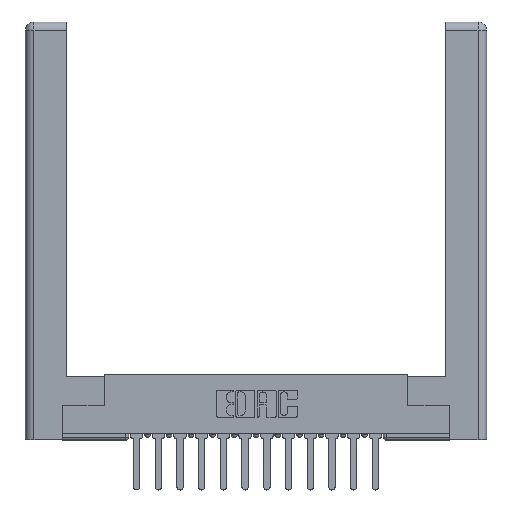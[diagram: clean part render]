
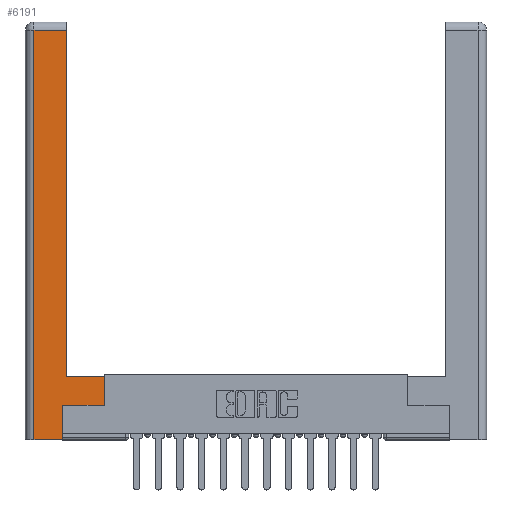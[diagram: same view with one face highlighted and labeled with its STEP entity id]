
A CAD part, top view. The second image highlights one B-rep face of the part: STEP entity #6191.
In plain terms, the highlighted planar face has unit normal (0, 0, 1).
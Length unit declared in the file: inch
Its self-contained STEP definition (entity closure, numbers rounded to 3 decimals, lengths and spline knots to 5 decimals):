
#5 = DIRECTION ( 'NONE',  ( -1., 0., 0. ) ) ;
#733 = LINE ( 'NONE', #2694, #1155 ) ;
#1034 = CARTESIAN_POINT ( 'NONE',  ( 0.565, 0.245, 0. ) ) ;
#1141 = DIRECTION ( 'NONE',  ( -1., 0., 0. ) ) ;
#1155 = VECTOR ( 'NONE', #15432, 39.37008 ) ;
#1436 = LINE ( 'NONE', #6506, #6390 ) ;
#1585 = VERTEX_POINT ( 'NONE', #7321 ) ;
#1708 = EDGE_CURVE ( 'NONE', #6962, #1585, #14943, .T. ) ;
#2441 = VERTEX_POINT ( 'NONE', #6844 ) ;
#2444 = CARTESIAN_POINT ( 'NONE',  ( 0.265, 0.245, 0. ) ) ;
#2694 = CARTESIAN_POINT ( 'NONE',  ( 0.295, 3., 0. ) ) ;
#2912 = EDGE_CURVE ( 'NONE', #2441, #9226, #13292, .T. ) ;
#3000 = CARTESIAN_POINT ( 'NONE',  ( 0.265, 0., 0. ) ) ;
#3029 = EDGE_CURVE ( 'NONE', #1585, #14190, #6334, .T. ) ;
#3034 = CARTESIAN_POINT ( 'NONE',  ( 0.565, 0.45, 0. ) ) ;
#3128 = LINE ( 'NONE', #3000, #5812 ) ;
#3150 = EDGE_CURVE ( 'NONE', #5322, #2441, #16774, .T. ) ;
#4112 = EDGE_CURVE ( 'NONE', #9226, #6962, #733, .T. ) ;
#4946 = CARTESIAN_POINT ( 'NONE',  ( 0.295, 0.45, 0. ) ) ;
#5085 = VECTOR ( 'NONE', #12213, 39.37008 ) ;
#5322 = VERTEX_POINT ( 'NONE', #12690 ) ;
#5392 = CARTESIAN_POINT ( 'NONE',  ( 0.0615, 2.94, 0. ) ) ;
#5812 = VECTOR ( 'NONE', #12168, 39.37008 ) ;
#6191 = ADVANCED_FACE ( 'NONE', ( #7408 ), #15549, .F. ) ;
#6334 = LINE ( 'NONE', #15908, #10617 ) ;
#6390 = VECTOR ( 'NONE', #15738, 39.37008 ) ;
#6506 = CARTESIAN_POINT ( 'NONE',  ( 0.265, 0.245, 0. ) ) ;
#6844 = CARTESIAN_POINT ( 'NONE',  ( 0.565, 0.45, 0. ) ) ;
#6962 = VERTEX_POINT ( 'NONE', #15810 ) ;
#7321 = CARTESIAN_POINT ( 'NONE',  ( 0.0615, 2.94, 0. ) ) ;
#7379 = ORIENTED_EDGE ( 'NONE', *, *, #2912, .T. ) ;
#7408 = FACE_OUTER_BOUND ( 'NONE', #9188, .T. ) ;
#7772 = VECTOR ( 'NONE', #5, 39.37008 ) ;
#8110 = CARTESIAN_POINT ( 'NONE',  ( 0.0615, 0., 0. ) ) ;
#8748 = VERTEX_POINT ( 'NONE', #10794 ) ;
#8951 = DIRECTION ( 'NONE',  ( 1., 0., 0. ) ) ;
#8994 = ORIENTED_EDGE ( 'NONE', *, *, #15772, .T. ) ;
#9058 = DIRECTION ( 'NONE',  ( 0., 0., -1. ) ) ;
#9188 = EDGE_LOOP ( 'NONE', ( #15374, #13847, #16824, #9579, #13241, #8994, #16793, #7379 ) ) ;
#9226 = VERTEX_POINT ( 'NONE', #4946 ) ;
#9579 = ORIENTED_EDGE ( 'NONE', *, *, #14899, .T. ) ;
#10500 = LINE ( 'NONE', #1034, #11727 ) ;
#10617 = VECTOR ( 'NONE', #11813, 39.37008 ) ;
#10751 = VERTEX_POINT ( 'NONE', #2444 ) ;
#10794 = CARTESIAN_POINT ( 'NONE',  ( 0.265, 0., 0. ) ) ;
#11226 = VECTOR ( 'NONE', #15627, 39.37008 ) ;
#11727 = VECTOR ( 'NONE', #8951, 39.37008 ) ;
#11813 = DIRECTION ( 'NONE',  ( 0., -1., 0. ) ) ;
#12168 = DIRECTION ( 'NONE',  ( 1., 0., 0. ) ) ;
#12213 = DIRECTION ( 'NONE',  ( 0., 1., 0. ) ) ;
#12690 = CARTESIAN_POINT ( 'NONE',  ( 0.565, 0.245, 0. ) ) ;
#13241 = ORIENTED_EDGE ( 'NONE', *, *, #16968, .T. ) ;
#13292 = LINE ( 'NONE', #16993, #11226 ) ;
#13847 = ORIENTED_EDGE ( 'NONE', *, *, #1708, .T. ) ;
#14190 = VERTEX_POINT ( 'NONE', #8110 ) ;
#14899 = EDGE_CURVE ( 'NONE', #14190, #8748, #3128, .T. ) ;
#14943 = LINE ( 'NONE', #5392, #7772 ) ;
#15205 = AXIS2_PLACEMENT_3D ( 'NONE', #16846, #9058, #1141 ) ;
#15374 = ORIENTED_EDGE ( 'NONE', *, *, #4112, .T. ) ;
#15432 = DIRECTION ( 'NONE',  ( 0., 1., 0. ) ) ;
#15549 = PLANE ( 'NONE',  #15205 ) ;
#15627 = DIRECTION ( 'NONE',  ( -1., 0., 0. ) ) ;
#15738 = DIRECTION ( 'NONE',  ( 0., 1., 0. ) ) ;
#15772 = EDGE_CURVE ( 'NONE', #10751, #5322, #10500, .T. ) ;
#15810 = CARTESIAN_POINT ( 'NONE',  ( 0.295, 2.94, 0. ) ) ;
#15908 = CARTESIAN_POINT ( 'NONE',  ( 0.0615, 0., 0. ) ) ;
#16774 = LINE ( 'NONE', #3034, #5085 ) ;
#16793 = ORIENTED_EDGE ( 'NONE', *, *, #3150, .T. ) ;
#16824 = ORIENTED_EDGE ( 'NONE', *, *, #3029, .T. ) ;
#16846 = CARTESIAN_POINT ( 'NONE',  ( 0., 0., 0. ) ) ;
#16968 = EDGE_CURVE ( 'NONE', #8748, #10751, #1436, .T. ) ;
#16993 = CARTESIAN_POINT ( 'NONE',  ( 0.295, 0.45, 0. ) ) ;
